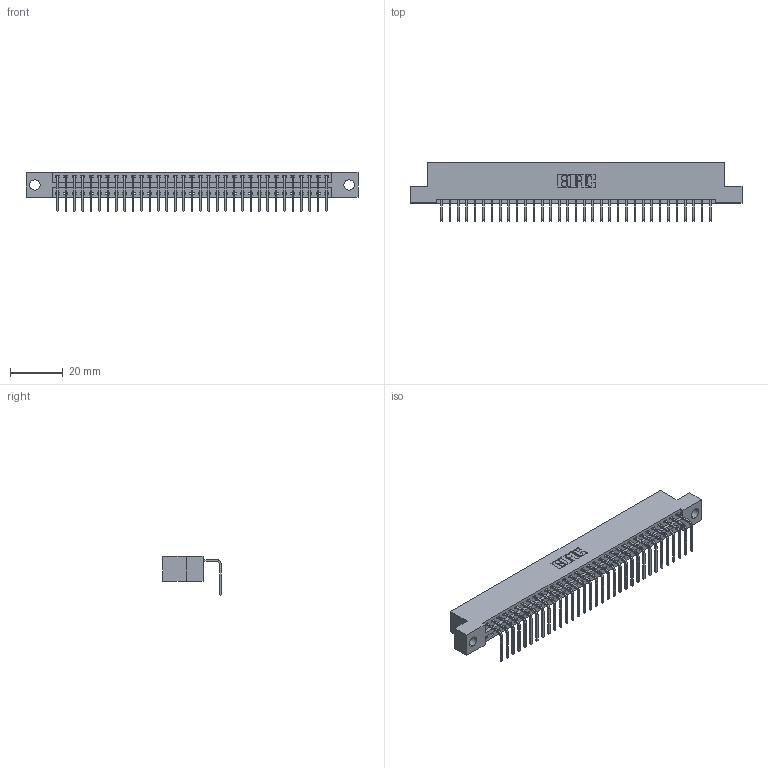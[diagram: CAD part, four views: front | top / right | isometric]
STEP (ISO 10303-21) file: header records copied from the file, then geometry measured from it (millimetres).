
FILE_DESCRIPTION (( 'STEP AP203' ), '1' );
FILE_NAME ('396-033-558-104.STEP', '2019-11-01T07:08:40', ( '' ), ( '' ), 'SwSTEP 2.0', 'SolidWorks 2016', '' );
FILE_SCHEMA (( 'CONFIG_CONTROL_DESIGN' ));
Length unit declared in the file: inch
Products named in the file (3): 346 Part_Flush Mounting Lugs - 0.156 Dia-TH; 345-292-001_558 Tail - 2; 396-033-558-104
Assembly tree (34 placements, depth 2):
  396-033-558-104
    346 Part_Flush Mounting Lugs - 0.156 Dia-TH
    345-292-001_558 Tail - 2  x33
Bounding box: 125.35 x 22.16 x 14.73 mm (x, y, z)
Volume: 11958.8 mm3; surface area: 15310.7 mm2
Topology: 34 solids, 34 shells, 2102 faces, 6335 edges, 4178 vertices
Faces by surface type: plane 1462, cylinder 640
Entity records: 21779 total; most frequent: CARTESIAN_POINT 3743, ORIENTED_EDGE 3710, DIRECTION 3313, EDGE_CURVE 1855, LINE 1591, VECTOR 1591, VERTEX_POINT 1234, AXIS2_PLACEMENT_3D 861
